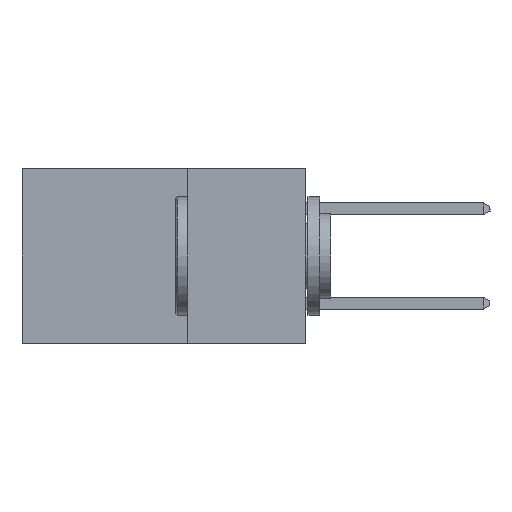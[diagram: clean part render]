
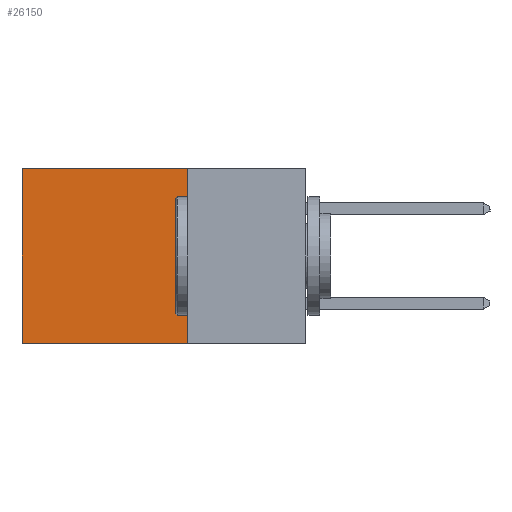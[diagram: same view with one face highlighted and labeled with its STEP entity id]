
A CAD part, left-side view. The second image highlights one B-rep face of the part: STEP entity #26150.
In plain terms, the highlighted planar face has unit normal (-1, 0, 0).
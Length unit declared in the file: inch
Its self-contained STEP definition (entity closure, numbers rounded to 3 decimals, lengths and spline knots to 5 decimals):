
#448 = AXIS2_PLACEMENT_3D ( 'NONE', #17573, #5534, #19592 ) ;
#2183 = FACE_OUTER_BOUND ( 'NONE', #15670, .T. ) ;
#2472 = CARTESIAN_POINT ( 'NONE',  ( 0.298, 0.25, 0. ) ) ;
#2551 = LINE ( 'NONE', #19467, #13305 ) ;
#3656 = CARTESIAN_POINT ( 'NONE',  ( 0.298, 0.6, -0.37 ) ) ;
#4334 = CARTESIAN_POINT ( 'NONE',  ( 0.298, 0.25, -0.37 ) ) ;
#4616 = DIRECTION ( 'NONE',  ( 0., 0., -1. ) ) ;
#5534 = DIRECTION ( 'NONE',  ( 1., 0., 0. ) ) ;
#5754 = CARTESIAN_POINT ( 'NONE',  ( 0.298, 0.6, 0. ) ) ;
#7101 = ORIENTED_EDGE ( 'NONE', *, *, #14630, .T. ) ;
#7413 = DIRECTION ( 'NONE',  ( 0., 1., 0. ) ) ;
#8511 = ORIENTED_EDGE ( 'NONE', *, *, #15339, .F. ) ;
#10165 = LINE ( 'NONE', #2472, #25527 ) ;
#10917 = LINE ( 'NONE', #22364, #21019 ) ;
#11441 = PLANE ( 'NONE',  #448 ) ;
#11907 = CARTESIAN_POINT ( 'NONE',  ( 0.298, 0.25, -0.37 ) ) ;
#13305 = VECTOR ( 'NONE', #7413, 39.37008 ) ;
#14630 = EDGE_CURVE ( 'NONE', #17999, #25687, #10917, .T. ) ;
#15082 = ORIENTED_EDGE ( 'NONE', *, *, #25563, .T. ) ;
#15339 = EDGE_CURVE ( 'NONE', #22837, #25687, #15967, .T. ) ;
#15670 = EDGE_LOOP ( 'NONE', ( #7101, #8511, #20721, #15082 ) ) ;
#15967 = LINE ( 'NONE', #4334, #21915 ) ;
#16549 = VERTEX_POINT ( 'NONE', #25372 ) ;
#17573 = CARTESIAN_POINT ( 'NONE',  ( 0.298, 0.25, 0. ) ) ;
#17999 = VERTEX_POINT ( 'NONE', #5754 ) ;
#18408 = DIRECTION ( 'NONE',  ( 0., 1., 0. ) ) ;
#19467 = CARTESIAN_POINT ( 'NONE',  ( 0.298, 0.25, 0. ) ) ;
#19592 = DIRECTION ( 'NONE',  ( 0., 0., -1. ) ) ;
#20721 = ORIENTED_EDGE ( 'NONE', *, *, #23365, .F. ) ;
#21019 = VECTOR ( 'NONE', #24338, 39.37008 ) ;
#21915 = VECTOR ( 'NONE', #18408, 39.37008 ) ;
#22364 = CARTESIAN_POINT ( 'NONE',  ( 0.298, 0.6, 0. ) ) ;
#22837 = VERTEX_POINT ( 'NONE', #11907 ) ;
#23365 = EDGE_CURVE ( 'NONE', #16549, #22837, #10165, .T. ) ;
#24338 = DIRECTION ( 'NONE',  ( 0., 0., -1. ) ) ;
#25372 = CARTESIAN_POINT ( 'NONE',  ( 0.298, 0.25, 0. ) ) ;
#25527 = VECTOR ( 'NONE', #4616, 39.37008 ) ;
#25563 = EDGE_CURVE ( 'NONE', #16549, #17999, #2551, .T. ) ;
#25687 = VERTEX_POINT ( 'NONE', #3656 ) ;
#26150 = ADVANCED_FACE ( 'NONE', ( #2183 ), #11441, .F. ) ;
